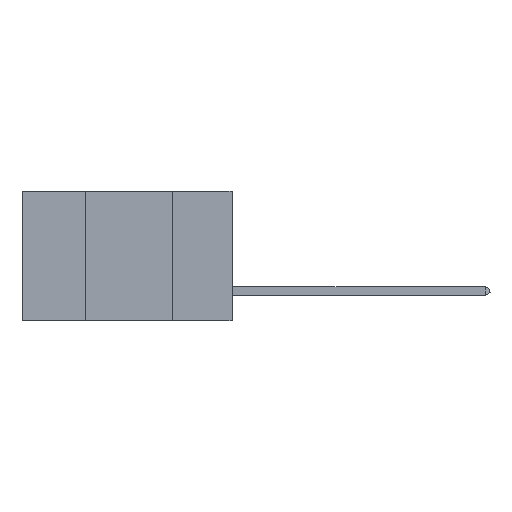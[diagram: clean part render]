
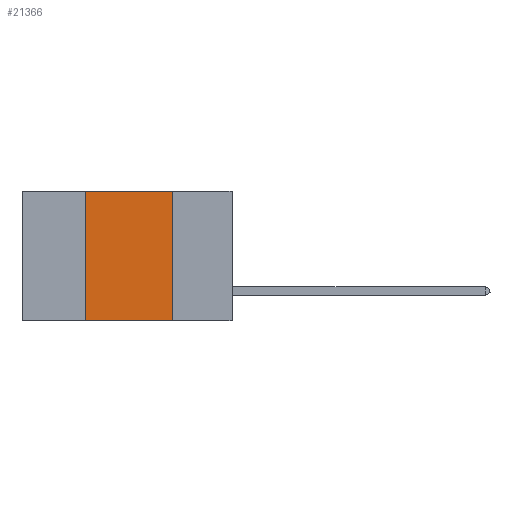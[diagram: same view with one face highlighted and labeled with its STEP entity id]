
A CAD part, left-side view. The second image highlights one B-rep face of the part: STEP entity #21366.
In plain terms, the highlighted planar face has unit normal (-1, 0, 0).
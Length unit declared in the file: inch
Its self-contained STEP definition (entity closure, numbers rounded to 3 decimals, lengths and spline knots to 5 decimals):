
#1205 = PLANE ( 'NONE',  #2410 ) ;
#1741 = CARTESIAN_POINT ( 'NONE',  ( 0., 0.6, 0. ) ) ;
#1792 = DIRECTION ( 'NONE',  ( 0., -1., 0. ) ) ;
#2177 = VERTEX_POINT ( 'NONE', #12639 ) ;
#2410 = AXIS2_PLACEMENT_3D ( 'NONE', #1741, #9279, #4320 ) ;
#2910 = VECTOR ( 'NONE', #11303, 39.37008 ) ;
#4320 = DIRECTION ( 'NONE',  ( 0., 0., -1. ) ) ;
#4855 = EDGE_LOOP ( 'NONE', ( #34947, #22034, #35268, #13254 ) ) ;
#5546 = EDGE_CURVE ( 'NONE', #2177, #21328, #11646, .T. ) ;
#6518 = CARTESIAN_POINT ( 'NONE',  ( 0., 0.17, 0. ) ) ;
#8471 = CARTESIAN_POINT ( 'NONE',  ( 0., 0.17, -0.37 ) ) ;
#9279 = DIRECTION ( 'NONE',  ( 1., 0., 0. ) ) ;
#9818 = VECTOR ( 'NONE', #13857, 39.37008 ) ;
#11303 = DIRECTION ( 'NONE',  ( 0., -1., 0. ) ) ;
#11646 = LINE ( 'NONE', #34259, #2910 ) ;
#12295 = VERTEX_POINT ( 'NONE', #8471 ) ;
#12405 = CARTESIAN_POINT ( 'NONE',  ( 0., 0.42, 0. ) ) ;
#12639 = CARTESIAN_POINT ( 'NONE',  ( 0., 0.42, 0. ) ) ;
#12761 = LINE ( 'NONE', #12405, #23527 ) ;
#13254 = ORIENTED_EDGE ( 'NONE', *, *, #14096, .T. ) ;
#13857 = DIRECTION ( 'NONE',  ( 0., 0., -1. ) ) ;
#13991 = VERTEX_POINT ( 'NONE', #20535 ) ;
#14096 = EDGE_CURVE ( 'NONE', #13991, #12295, #29354, .T. ) ;
#20483 = DIRECTION ( 'NONE',  ( 0., 0., 1. ) ) ;
#20535 = CARTESIAN_POINT ( 'NONE',  ( 0., 0.42, -0.37 ) ) ;
#21208 = FACE_OUTER_BOUND ( 'NONE', #4855, .T. ) ;
#21299 = EDGE_CURVE ( 'NONE', #13991, #2177, #12761, .T. ) ;
#21328 = VERTEX_POINT ( 'NONE', #6518 ) ;
#21366 = ADVANCED_FACE ( 'NONE', ( #21208 ), #1205, .F. ) ;
#22034 = ORIENTED_EDGE ( 'NONE', *, *, #5546, .F. ) ;
#23527 = VECTOR ( 'NONE', #20483, 39.37008 ) ;
#24343 = LINE ( 'NONE', #35560, #9818 ) ;
#27716 = VECTOR ( 'NONE', #1792, 39.37008 ) ;
#29354 = LINE ( 'NONE', #33190, #27716 ) ;
#33190 = CARTESIAN_POINT ( 'NONE',  ( 0., 0.6, -0.37 ) ) ;
#33235 = EDGE_CURVE ( 'NONE', #21328, #12295, #24343, .T. ) ;
#34259 = CARTESIAN_POINT ( 'NONE',  ( 0., 0.6, 0. ) ) ;
#34947 = ORIENTED_EDGE ( 'NONE', *, *, #33235, .F. ) ;
#35268 = ORIENTED_EDGE ( 'NONE', *, *, #21299, .F. ) ;
#35560 = CARTESIAN_POINT ( 'NONE',  ( 0., 0.17, 0. ) ) ;
